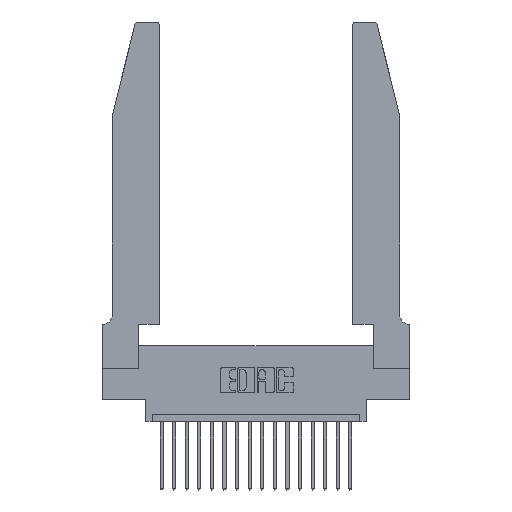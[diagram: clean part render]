
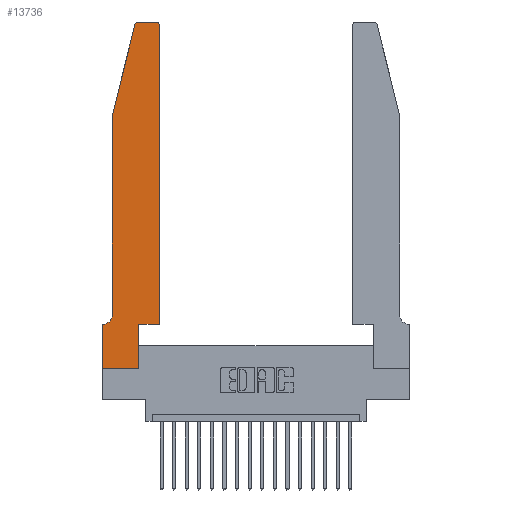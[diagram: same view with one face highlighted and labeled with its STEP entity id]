
A CAD part, top view. The second image highlights one B-rep face of the part: STEP entity #13736.
In plain terms, the highlighted planar face has unit normal (0, 0, 1).
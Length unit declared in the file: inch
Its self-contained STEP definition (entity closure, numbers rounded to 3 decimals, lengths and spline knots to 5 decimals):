
#170 = EDGE_CURVE ( 'NONE', #1734, #1491, #15143, .T. ) ;
#231 = LINE ( 'NONE', #1536, #15589 ) ;
#392 = DIRECTION ( 'NONE',  ( 0., 0., 1. ) ) ;
#563 = LINE ( 'NONE', #5975, #3749 ) ;
#677 = ORIENTED_EDGE ( 'NONE', *, *, #12100, .T. ) ;
#1285 = ORIENTED_EDGE ( 'NONE', *, *, #10059, .T. ) ;
#1491 = VERTEX_POINT ( 'NONE', #9969 ) ;
#1536 = CARTESIAN_POINT ( 'NONE',  ( 0.2605, 2.75, 0.37 ) ) ;
#1734 = VERTEX_POINT ( 'NONE', #11118 ) ;
#1777 = DIRECTION ( 'NONE',  ( 1., 0., 0. ) ) ;
#1981 = CARTESIAN_POINT ( 'NONE',  ( 0., 0., 0.37 ) ) ;
#1998 = DIRECTION ( 'NONE',  ( 1., 0., 0. ) ) ;
#2214 = CARTESIAN_POINT ( 'NONE',  ( 0.4205, 2.72, 0.37 ) ) ;
#2544 = AXIS2_PLACEMENT_3D ( 'NONE', #6169, #4476, #6249 ) ;
#2625 = EDGE_CURVE ( 'NONE', #5190, #6488, #16995, .T. ) ;
#2692 = EDGE_CURVE ( 'NONE', #6215, #1734, #5610, .T. ) ;
#2696 = ORIENTED_EDGE ( 'NONE', *, *, #2692, .T. ) ;
#2775 = CIRCLE ( 'NONE', #19975, 0.07 ) ;
#3032 = CARTESIAN_POINT ( 'NONE',  ( 0.2865, 0., 0.37 ) ) ;
#3061 = ORIENTED_EDGE ( 'NONE', *, *, #2625, .T. ) ;
#3471 = CARTESIAN_POINT ( 'NONE',  ( 0.0755, 2., 0.37 ) ) ;
#3490 = PLANE ( 'NONE',  #19201 ) ;
#3749 = VECTOR ( 'NONE', #18343, 39.37008 ) ;
#3776 = DIRECTION ( 'NONE',  ( 0., 0., 1. ) ) ;
#4476 = DIRECTION ( 'NONE',  ( 0., 0., 1. ) ) ;
#4503 = CARTESIAN_POINT ( 'NONE',  ( 0., 0., 0.37 ) ) ;
#5015 = DIRECTION ( 'NONE',  ( -1., 0., 0. ) ) ;
#5190 = VERTEX_POINT ( 'NONE', #12389 ) ;
#5311 = VERTEX_POINT ( 'NONE', #4503 ) ;
#5344 = EDGE_CURVE ( 'NONE', #15652, #8093, #2775, .T. ) ;
#5375 = ORIENTED_EDGE ( 'NONE', *, *, #9062, .T. ) ;
#5610 = LINE ( 'NONE', #6053, #7122 ) ;
#5686 = EDGE_CURVE ( 'NONE', #10342, #6827, #563, .T. ) ;
#5856 = CARTESIAN_POINT ( 'NONE',  ( 0.284, 2.75, 0.37 ) ) ;
#5975 = CARTESIAN_POINT ( 'NONE',  ( 0.0755, 2., 0.37 ) ) ;
#5976 = EDGE_LOOP ( 'NONE', ( #677, #7306, #12649, #16515, #11242, #1285, #11489, #18455, #2696, #15127, #5375, #3061 ) ) ;
#6053 = CARTESIAN_POINT ( 'NONE',  ( 0.2865, 0.35, 0.37 ) ) ;
#6169 = CARTESIAN_POINT ( 'NONE',  ( 0.284, 2.72, 0.37 ) ) ;
#6215 = VERTEX_POINT ( 'NONE', #3032 ) ;
#6249 = DIRECTION ( 'NONE',  ( 1., 0., 0. ) ) ;
#6293 = DIRECTION ( 'NONE',  ( 0., 0., -1. ) ) ;
#6488 = VERTEX_POINT ( 'NONE', #20281 ) ;
#6774 = CARTESIAN_POINT ( 'NONE',  ( 0., 0.35, 0.37 ) ) ;
#6827 = VERTEX_POINT ( 'NONE', #3471 ) ;
#6847 = CARTESIAN_POINT ( 'NONE',  ( 0.4505, 0.35, 0.37 ) ) ;
#7122 = VECTOR ( 'NONE', #13893, 39.37008 ) ;
#7306 = ORIENTED_EDGE ( 'NONE', *, *, #15726, .T. ) ;
#7338 = FACE_OUTER_BOUND ( 'NONE', #5976, .T. ) ;
#7481 = LINE ( 'NONE', #6847, #15909 ) ;
#7670 = VERTEX_POINT ( 'NONE', #15830 ) ;
#8080 = DIRECTION ( 'NONE',  ( 1., 0., 0. ) ) ;
#8093 = VERTEX_POINT ( 'NONE', #13300 ) ;
#8692 = CARTESIAN_POINT ( 'NONE',  ( 0., 0., 0.37 ) ) ;
#9062 = EDGE_CURVE ( 'NONE', #1491, #5190, #7481, .T. ) ;
#9334 = EDGE_CURVE ( 'NONE', #7670, #5311, #15174, .T. ) ;
#9681 = VECTOR ( 'NONE', #14095, 39.37008 ) ;
#9755 = CARTESIAN_POINT ( 'NONE',  ( 0.4505, 0.35, 0.37 ) ) ;
#9909 = LINE ( 'NONE', #1981, #16092 ) ;
#9947 = CARTESIAN_POINT ( 'NONE',  ( 0.25487, 2.72718, 0.37 ) ) ;
#9969 = CARTESIAN_POINT ( 'NONE',  ( 0.4505, 0.35, 0.37 ) ) ;
#10059 = EDGE_CURVE ( 'NONE', #8093, #7670, #12655, .T. ) ;
#10084 = DIRECTION ( 'NONE',  ( 0., 1., 0. ) ) ;
#10342 = VERTEX_POINT ( 'NONE', #9947 ) ;
#10944 = CARTESIAN_POINT ( 'NONE',  ( 0.0055, 0.42, 0.37 ) ) ;
#11118 = CARTESIAN_POINT ( 'NONE',  ( 0.2865, 0.35, 0.37 ) ) ;
#11242 = ORIENTED_EDGE ( 'NONE', *, *, #5344, .T. ) ;
#11438 = VECTOR ( 'NONE', #1998, 39.37008 ) ;
#11489 = ORIENTED_EDGE ( 'NONE', *, *, #9334, .T. ) ;
#11898 = AXIS2_PLACEMENT_3D ( 'NONE', #2214, #3776, #18026 ) ;
#12100 = EDGE_CURVE ( 'NONE', #6488, #16844, #231, .T. ) ;
#12389 = CARTESIAN_POINT ( 'NONE',  ( 0.4505, 2.72, 0.37 ) ) ;
#12649 = ORIENTED_EDGE ( 'NONE', *, *, #5686, .T. ) ;
#12655 = LINE ( 'NONE', #17158, #9681 ) ;
#12703 = CIRCLE ( 'NONE', #2544, 0.03 ) ;
#13300 = CARTESIAN_POINT ( 'NONE',  ( 0.0055, 0.35, 0.37 ) ) ;
#13736 = ADVANCED_FACE ( 'NONE', ( #7338 ), #3490, .T. ) ;
#13893 = DIRECTION ( 'NONE',  ( 0., 1., 0. ) ) ;
#13947 = LINE ( 'NONE', #17964, #18093 ) ;
#13955 = DIRECTION ( 'NONE',  ( -1., 0., 0. ) ) ;
#14095 = DIRECTION ( 'NONE',  ( -1., 0., 0. ) ) ;
#15020 = DIRECTION ( 'NONE',  ( 0., -1., 0. ) ) ;
#15127 = ORIENTED_EDGE ( 'NONE', *, *, #170, .T. ) ;
#15143 = LINE ( 'NONE', #9755, #11438 ) ;
#15174 = LINE ( 'NONE', #8692, #20327 ) ;
#15589 = VECTOR ( 'NONE', #13955, 39.37008 ) ;
#15652 = VERTEX_POINT ( 'NONE', #18814 ) ;
#15726 = EDGE_CURVE ( 'NONE', #16844, #10342, #12703, .T. ) ;
#15830 = CARTESIAN_POINT ( 'NONE',  ( 0., 0.35, 0.37 ) ) ;
#15909 = VECTOR ( 'NONE', #10084, 39.37008 ) ;
#16092 = VECTOR ( 'NONE', #8080, 39.37008 ) ;
#16515 = ORIENTED_EDGE ( 'NONE', *, *, #20261, .T. ) ;
#16844 = VERTEX_POINT ( 'NONE', #5856 ) ;
#16995 = CIRCLE ( 'NONE', #11898, 0.03 ) ;
#17158 = CARTESIAN_POINT ( 'NONE',  ( 0.0755, 0.35, 0.37 ) ) ;
#17160 = EDGE_CURVE ( 'NONE', #5311, #6215, #9909, .T. ) ;
#17964 = CARTESIAN_POINT ( 'NONE',  ( 0.0755, 2., 0.37 ) ) ;
#18026 = DIRECTION ( 'NONE',  ( 1., 0., 0. ) ) ;
#18093 = VECTOR ( 'NONE', #20040, 39.37008 ) ;
#18343 = DIRECTION ( 'NONE',  ( -0.239, -0.971, 0. ) ) ;
#18455 = ORIENTED_EDGE ( 'NONE', *, *, #17160, .T. ) ;
#18814 = CARTESIAN_POINT ( 'NONE',  ( 0.0755, 0.42, 0.37 ) ) ;
#19201 = AXIS2_PLACEMENT_3D ( 'NONE', #6774, #392, #1777 ) ;
#19975 = AXIS2_PLACEMENT_3D ( 'NONE', #10944, #6293, #5015 ) ;
#20040 = DIRECTION ( 'NONE',  ( 0., -1., 0. ) ) ;
#20261 = EDGE_CURVE ( 'NONE', #6827, #15652, #13947, .T. ) ;
#20281 = CARTESIAN_POINT ( 'NONE',  ( 0.4205, 2.75, 0.37 ) ) ;
#20327 = VECTOR ( 'NONE', #15020, 39.37008 ) ;
